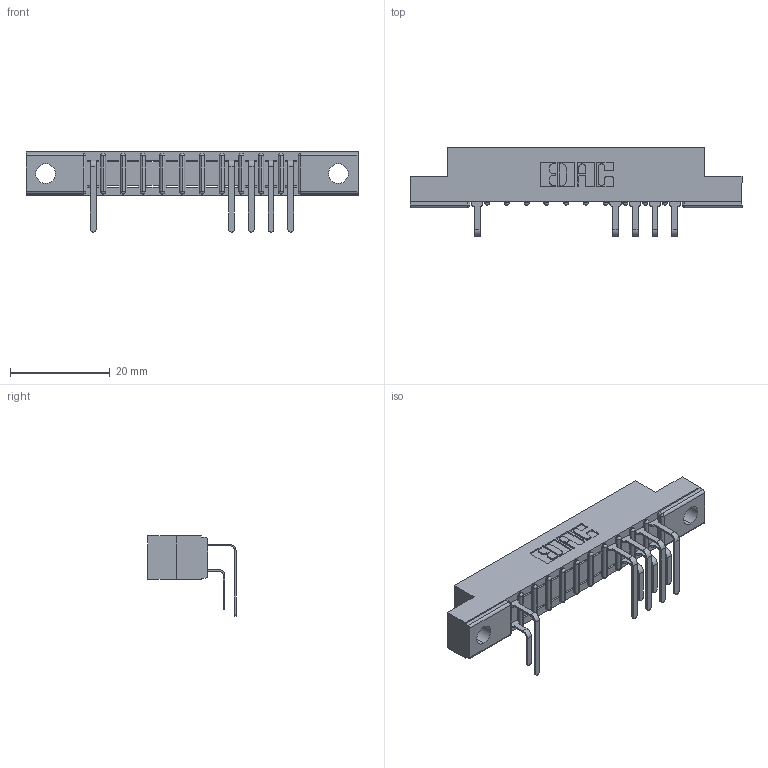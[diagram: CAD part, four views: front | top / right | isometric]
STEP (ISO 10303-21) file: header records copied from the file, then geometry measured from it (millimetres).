
FILE_DESCRIPTION (( 'STEP AP203' ), '1' );
FILE_NAME ('307-022-559-204.STEP', '2018-08-04T04:35:31', ( '' ), ( '' ), 'SwSTEP 2.0', 'SolidWorks 2016', '' );
FILE_SCHEMA (( 'CONFIG_CONTROL_DESIGN' ));
Length unit declared in the file: inch
Products named in the file (4): 307 Part_.156 Dia Mounting Holes; 307-290-001_558 559 - 1 (Single); 307-290-001_559 - 2 (Single); 307-022-559-204
Assembly tree (10 placements, depth 2):
  307-022-559-204
    307 Part_.156 Dia Mounting Holes
    307-290-001_558 559 - 1 (Single)  x4
    307-290-001_559 - 2 (Single)  x5
Bounding box: 66.6 x 17.69 x 16.08 mm (x, y, z)
Volume: 4124.8 mm3; surface area: 5840.8 mm2
Topology: 10 solids, 10 shells, 724 faces, 2053 edges, 1322 vertices
Faces by surface type: plane 459, cylinder 241, sphere 24
Entity records: 15053 total; most frequent: CARTESIAN_POINT 2534, ORIENTED_EDGE 2518, DIRECTION 2473, EDGE_CURVE 1259, LINE 959, VECTOR 959, VERTEX_POINT 818, AXIS2_PLACEMENT_3D 757
